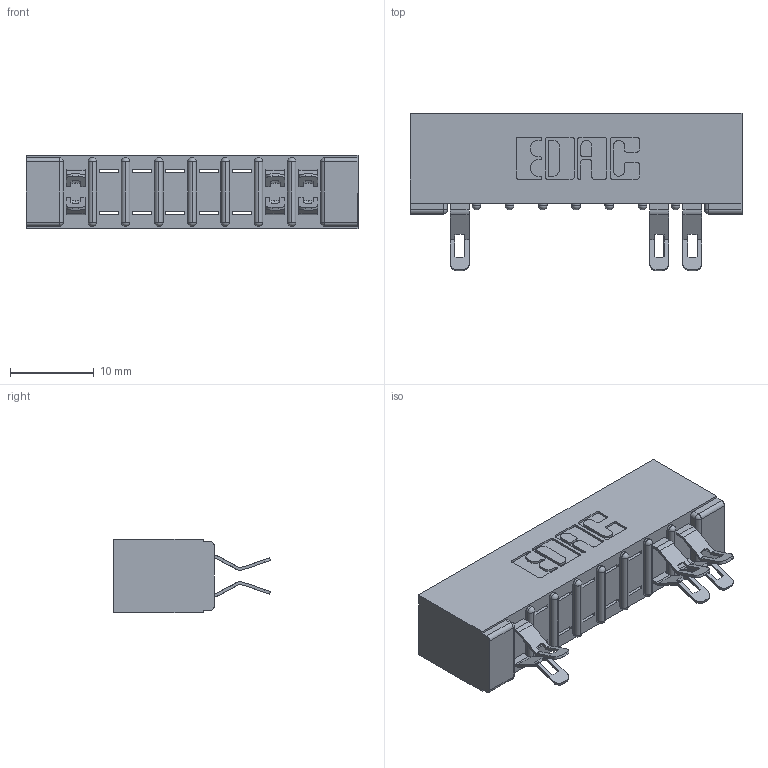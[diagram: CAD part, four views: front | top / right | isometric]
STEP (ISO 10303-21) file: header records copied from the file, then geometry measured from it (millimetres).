
FILE_DESCRIPTION (( 'STEP AP203' ), '1' );
FILE_NAME ('357-016-555-201.STEP', '2018-08-08T02:56:13', ( '' ), ( '' ), 'SwSTEP 2.0', 'SolidWorks 2016', '' );
FILE_SCHEMA (( 'CONFIG_CONTROL_DESIGN' ));
Length unit declared in the file: inch
Products named in the file (3): 307 Part_No Mounting Lugs; 307-290-001_555; 357-016-555-201
Assembly tree (7 placements, depth 2):
  357-016-555-201
    307 Part_No Mounting Lugs
    307-290-001_555  x6
Bounding box: 39.57 x 18.75 x 8.71 mm (x, y, z)
Volume: 2711.6 mm3; surface area: 3864.1 mm2
Topology: 7 solids, 7 shells, 585 faces, 1705 edges, 1102 vertices
Faces by surface type: plane 330, cylinder 237, sphere 18
Entity records: 11245 total; most frequent: CARTESIAN_POINT 1894, ORIENTED_EDGE 1884, DIRECTION 1866, EDGE_CURVE 942, VECTOR 698, LINE 698, VERTEX_POINT 612, AXIS2_PLACEMENT_3D 584
